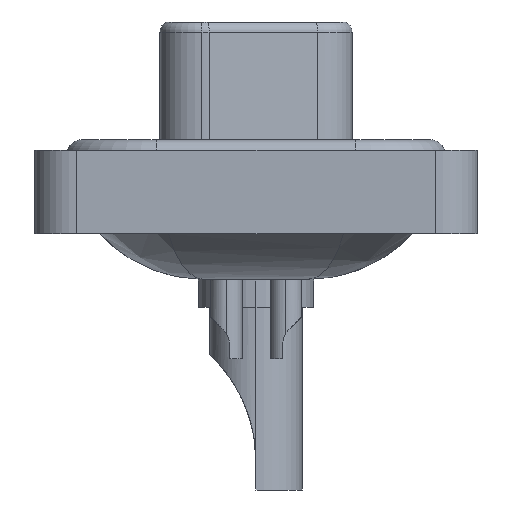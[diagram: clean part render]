
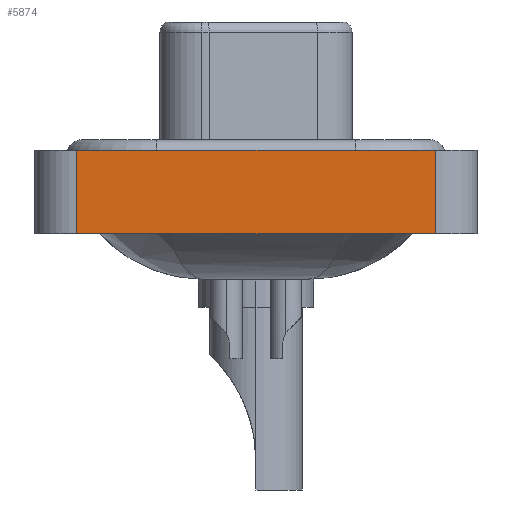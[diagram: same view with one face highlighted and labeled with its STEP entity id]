
A CAD part, left-side view. The second image highlights one B-rep face of the part: STEP entity #5874.
In plain terms, the highlighted planar face has unit normal (-1, 0, 0).
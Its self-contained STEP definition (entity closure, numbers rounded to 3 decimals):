
#485 = EDGE_CURVE ( 'NONE', #3835, #8307, #14616, .T. ) ;
#638 = CARTESIAN_POINT ( 'NONE',  ( -7.25, 8.55, -3.6 ) ) ;
#1047 = VECTOR ( 'NONE', #13830, 1000. ) ;
#2093 = DIRECTION ( 'NONE',  ( 0., 0., 1. ) ) ;
#2320 = LINE ( 'NONE', #10815, #1047 ) ;
#2375 = DIRECTION ( 'NONE',  ( 0., 0., 1. ) ) ;
#2497 = EDGE_CURVE ( 'NONE', #10149, #13416, #2320, .T. ) ;
#3570 = CARTESIAN_POINT ( 'NONE',  ( -7.25, -8.55, -3.6 ) ) ;
#3835 = VERTEX_POINT ( 'NONE', #638 ) ;
#3887 = CARTESIAN_POINT ( 'NONE',  ( -7.25, -8.55, -3.6 ) ) ;
#5507 = EDGE_CURVE ( 'NONE', #8307, #13416, #17749, .T. ) ;
#5874 = ADVANCED_FACE ( 'NONE', ( #11959 ), #13511, .T. ) ;
#6916 = ORIENTED_EDGE ( 'NONE', *, *, #5507, .T. ) ;
#8307 = VERTEX_POINT ( 'NONE', #3887 ) ;
#9877 = ORIENTED_EDGE ( 'NONE', *, *, #485, .T. ) ;
#10017 = VECTOR ( 'NONE', #2093, 1000. ) ;
#10149 = VERTEX_POINT ( 'NONE', #10970 ) ;
#10527 = VECTOR ( 'NONE', #2375, 1000. ) ;
#10591 = LINE ( 'NONE', #14704, #10017 ) ;
#10815 = CARTESIAN_POINT ( 'NONE',  ( -7.25, -8.55, 0.4 ) ) ;
#10970 = CARTESIAN_POINT ( 'NONE',  ( -7.25, 8.55, 0.4 ) ) ;
#11606 = VECTOR ( 'NONE', #17554, 1000. ) ;
#11959 = FACE_OUTER_BOUND ( 'NONE', #14202, .T. ) ;
#12023 = ORIENTED_EDGE ( 'NONE', *, *, #2497, .F. ) ;
#12446 = AXIS2_PLACEMENT_3D ( 'NONE', #13325, #16429, #14781 ) ;
#12627 = CARTESIAN_POINT ( 'NONE',  ( -7.25, -8.55, 0.4 ) ) ;
#13325 = CARTESIAN_POINT ( 'NONE',  ( -7.25, -8.55, -3.6 ) ) ;
#13416 = VERTEX_POINT ( 'NONE', #12627 ) ;
#13511 = PLANE ( 'NONE',  #12446 ) ;
#13830 = DIRECTION ( 'NONE',  ( 0., -1., 0. ) ) ;
#14014 = ORIENTED_EDGE ( 'NONE', *, *, #14319, .F. ) ;
#14202 = EDGE_LOOP ( 'NONE', ( #6916, #12023, #14014, #9877 ) ) ;
#14319 = EDGE_CURVE ( 'NONE', #3835, #10149, #10591, .T. ) ;
#14616 = LINE ( 'NONE', #14887, #11606 ) ;
#14704 = CARTESIAN_POINT ( 'NONE',  ( -7.25, 8.55, -3.6 ) ) ;
#14781 = DIRECTION ( 'NONE',  ( 0., 0., 1. ) ) ;
#14887 = CARTESIAN_POINT ( 'NONE',  ( -7.25, -8.55, -3.6 ) ) ;
#16429 = DIRECTION ( 'NONE',  ( -1., 0., 0. ) ) ;
#17554 = DIRECTION ( 'NONE',  ( 0., -1., 0. ) ) ;
#17749 = LINE ( 'NONE', #3570, #10527 ) ;
